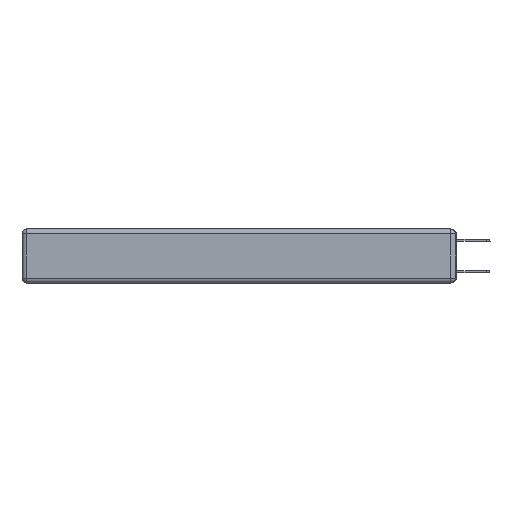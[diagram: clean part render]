
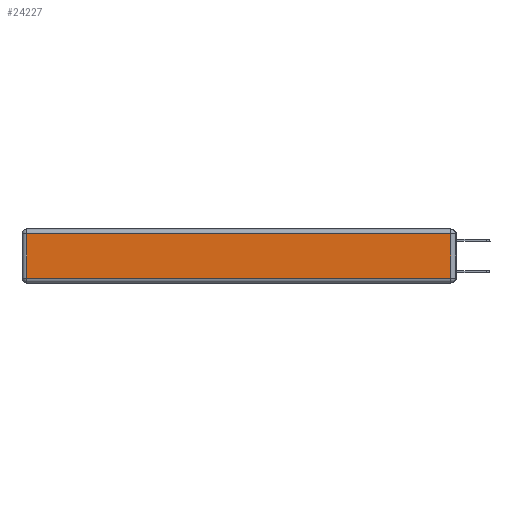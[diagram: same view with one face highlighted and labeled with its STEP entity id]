
A CAD part, left-side view. The second image highlights one B-rep face of the part: STEP entity #24227.
In plain terms, the highlighted planar face has unit normal (-1, 0, 0).
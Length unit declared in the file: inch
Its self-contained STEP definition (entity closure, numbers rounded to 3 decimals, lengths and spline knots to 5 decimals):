
#83 = EDGE_CURVE ( 'NONE', #18097, #707, #22492, .T. ) ;
#707 = VERTEX_POINT ( 'NONE', #2299 ) ;
#797 = VECTOR ( 'NONE', #18647, 39.37008 ) ;
#1392 = DIRECTION ( 'NONE',  ( 0., 0., -1. ) ) ;
#2008 = EDGE_CURVE ( 'NONE', #12073, #9081, #2161, .T. ) ;
#2161 = LINE ( 'NONE', #24786, #26865 ) ;
#2299 = CARTESIAN_POINT ( 'NONE',  ( 0., 2.72, -0.313 ) ) ;
#2436 = DIRECTION ( 'NONE',  ( 0., 0., 1. ) ) ;
#3987 = DIRECTION ( 'NONE',  ( -1., 0., 0. ) ) ;
#4093 = CARTESIAN_POINT ( 'NONE',  ( 0., 0., -0.313 ) ) ;
#4669 = EDGE_CURVE ( 'NONE', #9081, #18097, #7952, .T. ) ;
#6860 = EDGE_LOOP ( 'NONE', ( #19155, #24306, #26698, #13601 ) ) ;
#7952 = LINE ( 'NONE', #16326, #11484 ) ;
#9081 = VERTEX_POINT ( 'NONE', #9741 ) ;
#9741 = CARTESIAN_POINT ( 'NONE',  ( 0., 0.03, -0.03 ) ) ;
#10700 = CARTESIAN_POINT ( 'NONE',  ( 0., 0., -0.343 ) ) ;
#11484 = VECTOR ( 'NONE', #14252, 39.37008 ) ;
#12073 = VERTEX_POINT ( 'NONE', #23983 ) ;
#13601 = ORIENTED_EDGE ( 'NONE', *, *, #83, .T. ) ;
#13871 = CARTESIAN_POINT ( 'NONE',  ( 0., 2.72, -0.343 ) ) ;
#14252 = DIRECTION ( 'NONE',  ( 0., 1., 0. ) ) ;
#16326 = CARTESIAN_POINT ( 'NONE',  ( 0., 2.75, -0.03 ) ) ;
#16611 = AXIS2_PLACEMENT_3D ( 'NONE', #10700, #3987, #20710 ) ;
#17746 = EDGE_CURVE ( 'NONE', #707, #12073, #25318, .T. ) ;
#18097 = VERTEX_POINT ( 'NONE', #26679 ) ;
#18301 = VECTOR ( 'NONE', #1392, 39.37008 ) ;
#18647 = DIRECTION ( 'NONE',  ( 0., -1., 0. ) ) ;
#19155 = ORIENTED_EDGE ( 'NONE', *, *, #17746, .T. ) ;
#20710 = DIRECTION ( 'NONE',  ( 0., 0., 1. ) ) ;
#21105 = PLANE ( 'NONE',  #16611 ) ;
#22492 = LINE ( 'NONE', #13871, #18301 ) ;
#23983 = CARTESIAN_POINT ( 'NONE',  ( 0., 0.03, -0.313 ) ) ;
#24227 = ADVANCED_FACE ( 'NONE', ( #25100 ), #21105, .T. ) ;
#24306 = ORIENTED_EDGE ( 'NONE', *, *, #2008, .T. ) ;
#24786 = CARTESIAN_POINT ( 'NONE',  ( 0., 0.03, -0.343 ) ) ;
#25100 = FACE_OUTER_BOUND ( 'NONE', #6860, .T. ) ;
#25318 = LINE ( 'NONE', #4093, #797 ) ;
#26679 = CARTESIAN_POINT ( 'NONE',  ( 0., 2.72, -0.03 ) ) ;
#26698 = ORIENTED_EDGE ( 'NONE', *, *, #4669, .T. ) ;
#26865 = VECTOR ( 'NONE', #2436, 39.37008 ) ;
